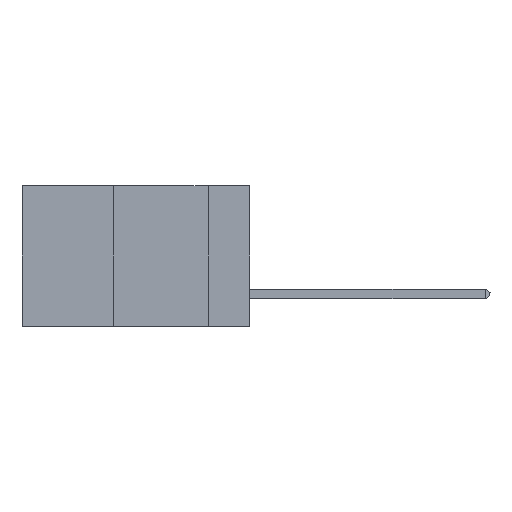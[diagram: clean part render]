
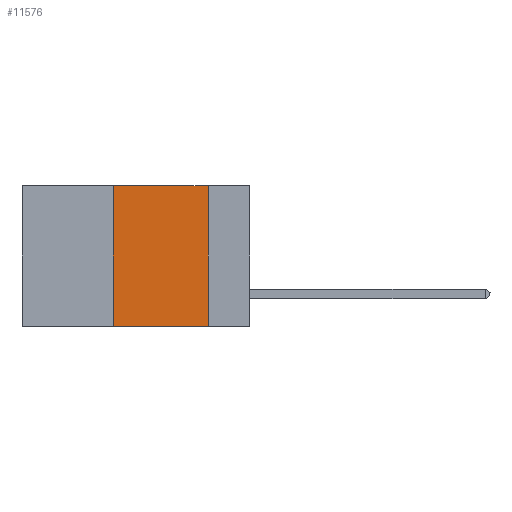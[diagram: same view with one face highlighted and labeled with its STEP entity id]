
A CAD part, left-side view. The second image highlights one B-rep face of the part: STEP entity #11576.
In plain terms, the highlighted planar face has unit normal (-1, 0, 0).
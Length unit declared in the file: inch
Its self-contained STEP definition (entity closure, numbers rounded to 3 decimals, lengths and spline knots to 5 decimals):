
#1037 = EDGE_LOOP ( 'NONE', ( #40182, #31113, #20773, #38401 ) ) ;
#2914 = EDGE_CURVE ( 'NONE', #37729, #28614, #30595, .T. ) ;
#3665 = LINE ( 'NONE', #23639, #24845 ) ;
#7116 = DIRECTION ( 'NONE',  ( 0., -1., 0. ) ) ;
#8193 = AXIS2_PLACEMENT_3D ( 'NONE', #37536, #17807, #21091 ) ;
#9627 = CARTESIAN_POINT ( 'NONE',  ( 0., 0.11, 0. ) ) ;
#9677 = CARTESIAN_POINT ( 'NONE',  ( 0., 0.36, 0. ) ) ;
#11576 = ADVANCED_FACE ( 'NONE', ( #30089 ), #34315, .F. ) ;
#12759 = LINE ( 'NONE', #9627, #23800 ) ;
#13242 = CARTESIAN_POINT ( 'NONE',  ( 0., 0.6, 0. ) ) ;
#14400 = VECTOR ( 'NONE', #20152, 39.37008 ) ;
#15921 = EDGE_CURVE ( 'NONE', #28614, #27756, #23121, .T. ) ;
#17280 = EDGE_CURVE ( 'NONE', #37729, #29131, #3665, .T. ) ;
#17807 = DIRECTION ( 'NONE',  ( 1., 0., 0. ) ) ;
#20152 = DIRECTION ( 'NONE',  ( 0., 0., 1. ) ) ;
#20773 = ORIENTED_EDGE ( 'NONE', *, *, #2914, .F. ) ;
#21091 = DIRECTION ( 'NONE',  ( 0., 0., -1. ) ) ;
#22681 = VECTOR ( 'NONE', #7116, 39.37008 ) ;
#23121 = LINE ( 'NONE', #13242, #22681 ) ;
#23639 = CARTESIAN_POINT ( 'NONE',  ( 0., 0.6, -0.37 ) ) ;
#23800 = VECTOR ( 'NONE', #35093, 39.37008 ) ;
#24845 = VECTOR ( 'NONE', #31712, 39.37008 ) ;
#27756 = VERTEX_POINT ( 'NONE', #38023 ) ;
#28614 = VERTEX_POINT ( 'NONE', #35326 ) ;
#29131 = VERTEX_POINT ( 'NONE', #32752 ) ;
#30089 = FACE_OUTER_BOUND ( 'NONE', #1037, .T. ) ;
#30595 = LINE ( 'NONE', #9677, #14400 ) ;
#31113 = ORIENTED_EDGE ( 'NONE', *, *, #15921, .F. ) ;
#31712 = DIRECTION ( 'NONE',  ( 0., -1., 0. ) ) ;
#32696 = CARTESIAN_POINT ( 'NONE',  ( 0., 0.36, -0.37 ) ) ;
#32752 = CARTESIAN_POINT ( 'NONE',  ( 0., 0.11, -0.37 ) ) ;
#34315 = PLANE ( 'NONE',  #8193 ) ;
#35093 = DIRECTION ( 'NONE',  ( 0., 0., -1. ) ) ;
#35326 = CARTESIAN_POINT ( 'NONE',  ( 0., 0.36, 0. ) ) ;
#36091 = EDGE_CURVE ( 'NONE', #27756, #29131, #12759, .T. ) ;
#37536 = CARTESIAN_POINT ( 'NONE',  ( 0., 0.6, 0. ) ) ;
#37729 = VERTEX_POINT ( 'NONE', #32696 ) ;
#38023 = CARTESIAN_POINT ( 'NONE',  ( 0., 0.11, 0. ) ) ;
#38401 = ORIENTED_EDGE ( 'NONE', *, *, #17280, .T. ) ;
#40182 = ORIENTED_EDGE ( 'NONE', *, *, #36091, .F. ) ;
